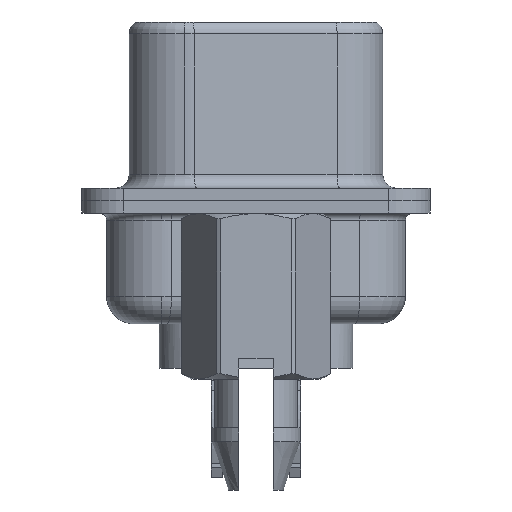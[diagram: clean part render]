
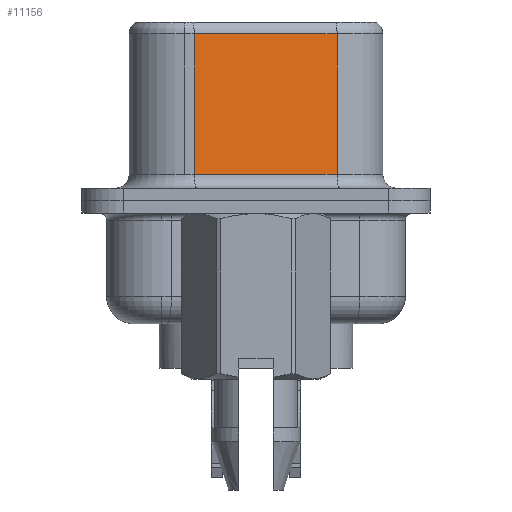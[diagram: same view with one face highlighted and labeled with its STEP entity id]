
A CAD part, left-side view. The second image highlights one B-rep face of the part: STEP entity #11156.
In plain terms, the highlighted planar face has unit normal (-0.985, -0.174, 0).
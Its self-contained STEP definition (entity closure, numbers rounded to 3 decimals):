
#530 = EDGE_LOOP ( 'NONE', ( #17990, #13996, #14489, #2373 ) ) ;
#721 = EDGE_CURVE ( 'NONE', #2652, #820, #15084, .T. ) ;
#820 = VERTEX_POINT ( 'NONE', #4431 ) ;
#1017 = CARTESIAN_POINT ( 'NONE',  ( 3.665, 2.233, 6.02 ) ) ;
#1024 = VERTEX_POINT ( 'NONE', #1017 ) ;
#2373 = ORIENTED_EDGE ( 'NONE', *, *, #11417, .T. ) ;
#2509 = CARTESIAN_POINT ( 'NONE',  ( 4.575, -2.927, 6.52 ) ) ;
#2652 = VERTEX_POINT ( 'NONE', #4813 ) ;
#2778 = DIRECTION ( 'NONE',  ( 0.174, -0.985, 0. ) ) ;
#3210 = EDGE_CURVE ( 'NONE', #2652, #1024, #14641, .T. ) ;
#3441 = CARTESIAN_POINT ( 'NONE',  ( 4.575, -2.927, 6.02 ) ) ;
#4431 = CARTESIAN_POINT ( 'NONE',  ( 4.575, -2.927, 0.95 ) ) ;
#4554 = CARTESIAN_POINT ( 'NONE',  ( 4.575, -2.927, 6.52 ) ) ;
#4813 = CARTESIAN_POINT ( 'NONE',  ( 4.575, -2.927, 6.02 ) ) ;
#6016 = DIRECTION ( 'NONE',  ( 0.985, 0.174, 0. ) ) ;
#6114 = FACE_OUTER_BOUND ( 'NONE', #530, .T. ) ;
#6637 = VECTOR ( 'NONE', #9038, 1000. ) ;
#9038 = DIRECTION ( 'NONE',  ( -0.174, 0.985, 0. ) ) ;
#10155 = DIRECTION ( 'NONE',  ( -0.174, 0.985, 0. ) ) ;
#10461 = VECTOR ( 'NONE', #15498, 1000. ) ;
#11137 = LINE ( 'NONE', #16726, #17692 ) ;
#11156 = ADVANCED_FACE ( 'NONE', ( #6114 ), #11529, .F. ) ;
#11417 = EDGE_CURVE ( 'NONE', #17251, #820, #11137, .T. ) ;
#11529 = PLANE ( 'NONE',  #17090 ) ;
#13183 = VECTOR ( 'NONE', #15354, 1000. ) ;
#13996 = ORIENTED_EDGE ( 'NONE', *, *, #3210, .T. ) ;
#14031 = LINE ( 'NONE', #15323, #10461 ) ;
#14489 = ORIENTED_EDGE ( 'NONE', *, *, #15428, .T. ) ;
#14641 = LINE ( 'NONE', #3441, #6637 ) ;
#15084 = LINE ( 'NONE', #2509, #13183 ) ;
#15323 = CARTESIAN_POINT ( 'NONE',  ( 3.665, 2.233, 6.52 ) ) ;
#15354 = DIRECTION ( 'NONE',  ( 0., 0., -1. ) ) ;
#15428 = EDGE_CURVE ( 'NONE', #1024, #17251, #14031, .T. ) ;
#15498 = DIRECTION ( 'NONE',  ( 0., 0., -1. ) ) ;
#16726 = CARTESIAN_POINT ( 'NONE',  ( 4.575, -2.927, 0.95 ) ) ;
#17090 = AXIS2_PLACEMENT_3D ( 'NONE', #4554, #6016, #10155 ) ;
#17251 = VERTEX_POINT ( 'NONE', #17590 ) ;
#17590 = CARTESIAN_POINT ( 'NONE',  ( 3.665, 2.233, 0.95 ) ) ;
#17692 = VECTOR ( 'NONE', #2778, 1000. ) ;
#17990 = ORIENTED_EDGE ( 'NONE', *, *, #721, .F. ) ;
